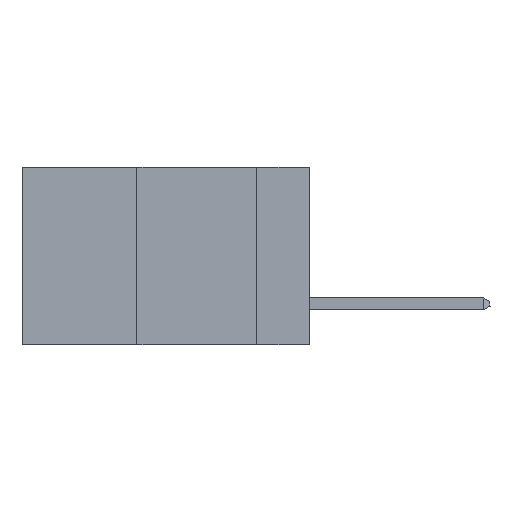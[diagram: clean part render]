
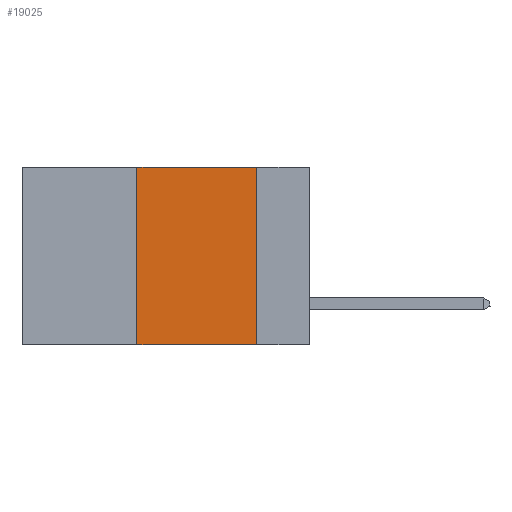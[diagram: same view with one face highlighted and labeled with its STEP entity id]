
A CAD part, left-side view. The second image highlights one B-rep face of the part: STEP entity #19025.
In plain terms, the highlighted planar face has unit normal (-1, 0, 0).
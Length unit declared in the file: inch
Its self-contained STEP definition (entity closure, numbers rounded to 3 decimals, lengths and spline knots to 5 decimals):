
#1031 = DIRECTION ( 'NONE',  ( 0., 0., -1. ) ) ;
#1396 = VERTEX_POINT ( 'NONE', #17636 ) ;
#1875 = DIRECTION ( 'NONE',  ( 0., -1., 0. ) ) ;
#2454 = EDGE_CURVE ( 'NONE', #1396, #11833, #8999, .T. ) ;
#2856 = VERTEX_POINT ( 'NONE', #15896 ) ;
#3378 = VECTOR ( 'NONE', #1031, 39.37008 ) ;
#3468 = VECTOR ( 'NONE', #1875, 39.37008 ) ;
#3555 = CARTESIAN_POINT ( 'NONE',  ( 0., 0.6, -0.37 ) ) ;
#4314 = EDGE_LOOP ( 'NONE', ( #7464, #17393, #20218, #14222 ) ) ;
#6157 = DIRECTION ( 'NONE',  ( 0., 0., -1. ) ) ;
#6281 = PLANE ( 'NONE',  #10751 ) ;
#6512 = EDGE_CURVE ( 'NONE', #14228, #2856, #10003, .T. ) ;
#6904 = FACE_OUTER_BOUND ( 'NONE', #4314, .T. ) ;
#7216 = VECTOR ( 'NONE', #9699, 39.37008 ) ;
#7464 = ORIENTED_EDGE ( 'NONE', *, *, #2454, .F. ) ;
#7712 = EDGE_CURVE ( 'NONE', #2856, #1396, #17912, .T. ) ;
#8470 = VECTOR ( 'NONE', #18972, 39.37008 ) ;
#8595 = CARTESIAN_POINT ( 'NONE',  ( 0., 0.11, 0. ) ) ;
#8803 = CARTESIAN_POINT ( 'NONE',  ( 0., 0.11, -0.37 ) ) ;
#8999 = LINE ( 'NONE', #8595, #3378 ) ;
#9134 = CARTESIAN_POINT ( 'NONE',  ( 0., 0.6, 0. ) ) ;
#9699 = DIRECTION ( 'NONE',  ( 0., -1., 0. ) ) ;
#10003 = LINE ( 'NONE', #14211, #8470 ) ;
#10751 = AXIS2_PLACEMENT_3D ( 'NONE', #9134, #20420, #6157 ) ;
#11833 = VERTEX_POINT ( 'NONE', #8803 ) ;
#14086 = LINE ( 'NONE', #3555, #3468 ) ;
#14211 = CARTESIAN_POINT ( 'NONE',  ( 0., 0.36, 0. ) ) ;
#14222 = ORIENTED_EDGE ( 'NONE', *, *, #18783, .T. ) ;
#14228 = VERTEX_POINT ( 'NONE', #18854 ) ;
#14427 = CARTESIAN_POINT ( 'NONE',  ( 0., 0.6, 0. ) ) ;
#15896 = CARTESIAN_POINT ( 'NONE',  ( 0., 0.36, 0. ) ) ;
#17393 = ORIENTED_EDGE ( 'NONE', *, *, #7712, .F. ) ;
#17636 = CARTESIAN_POINT ( 'NONE',  ( 0., 0.11, 0. ) ) ;
#17912 = LINE ( 'NONE', #14427, #7216 ) ;
#18783 = EDGE_CURVE ( 'NONE', #14228, #11833, #14086, .T. ) ;
#18854 = CARTESIAN_POINT ( 'NONE',  ( 0., 0.36, -0.37 ) ) ;
#18972 = DIRECTION ( 'NONE',  ( 0., 0., 1. ) ) ;
#19025 = ADVANCED_FACE ( 'NONE', ( #6904 ), #6281, .F. ) ;
#20218 = ORIENTED_EDGE ( 'NONE', *, *, #6512, .F. ) ;
#20420 = DIRECTION ( 'NONE',  ( 1., 0., 0. ) ) ;
